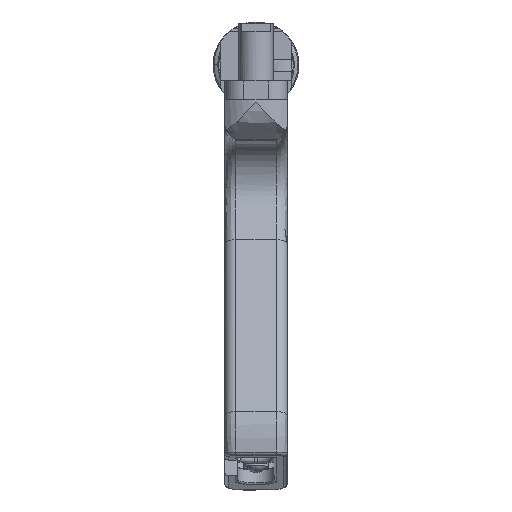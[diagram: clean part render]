
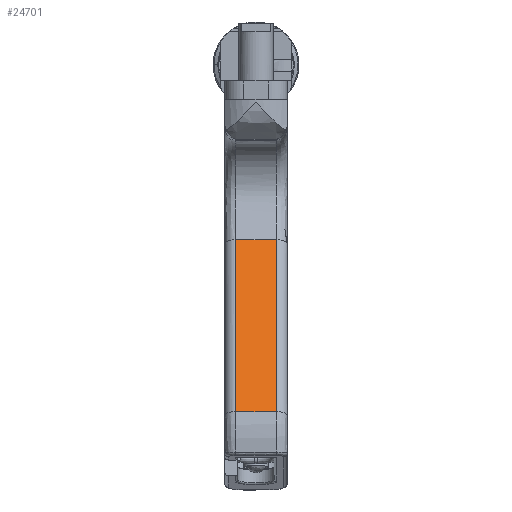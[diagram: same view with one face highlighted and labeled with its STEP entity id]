
A CAD part, front view. The second image highlights one B-rep face of the part: STEP entity #24701.
In plain terms, the highlighted planar face has unit normal (0, -0.902, 0.431).
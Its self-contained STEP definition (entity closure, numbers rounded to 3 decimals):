
#928=FACE_OUTER_BOUND('',#2314,.T.);
#2314=EDGE_LOOP('',(#17917,#17918,#17919,#17920));
#4368=LINE('',#35956,#7477);
#4582=LINE('',#37263,#7691);
#4584=LINE('',#37635,#7693);
#4585=LINE('',#37636,#7694);
#7477=VECTOR('',#28682,10.);
#7691=VECTOR('',#29244,10.);
#7693=VECTOR('',#29248,10.);
#7694=VECTOR('',#29249,10.);
#10550=VERTEX_POINT('',#35810);
#10551=VERTEX_POINT('',#35912);
#10752=VERTEX_POINT('',#37261);
#10753=VERTEX_POINT('',#37262);
#13146=EDGE_CURVE('',#10550,#10551,#4368,.T.);
#13468=EDGE_CURVE('',#10752,#10753,#4582,.T.);
#13474=EDGE_CURVE('',#10753,#10551,#4584,.T.);
#13475=EDGE_CURVE('',#10550,#10752,#4585,.T.);
#17917=ORIENTED_EDGE('',*,*,#13146,.T.);
#17918=ORIENTED_EDGE('',*,*,#13474,.F.);
#17919=ORIENTED_EDGE('',*,*,#13468,.F.);
#17920=ORIENTED_EDGE('',*,*,#13475,.F.);
#23492=PLANE('',#26274);
#24701=ADVANCED_FACE('',(#928),#23492,.T.);
#26274=AXIS2_PLACEMENT_3D('',#37634,#29246,#29247);
#28682=DIRECTION('',(1.,0.,0.));
#29244=DIRECTION('',(1.,0.,0.));
#29246=DIRECTION('center_axis',(0.,-0.902,0.431));
#29247=DIRECTION('ref_axis',(0.,-0.431,-0.902));
#29248=DIRECTION('',(0.,-0.431,-0.902));
#29249=DIRECTION('',(0.,0.431,0.902));
#35810=CARTESIAN_POINT('',(-5.414,-123.151,-44.136));
#35912=CARTESIAN_POINT('',(5.414,-123.151,-44.136));
#35956=CARTESIAN_POINT('',(0.,-123.151,-44.136));
#37261=CARTESIAN_POINT('',(-5.414,-101.106,2.016));
#37262=CARTESIAN_POINT('',(5.414,-101.106,2.016));
#37263=CARTESIAN_POINT('',(0.,-101.106,2.016));
#37634=CARTESIAN_POINT('Origin',(0.,-101.106,2.016));
#37635=CARTESIAN_POINT('',(5.414,-97.368,9.842));
#37636=CARTESIAN_POINT('',(-5.414,-97.368,9.842));
